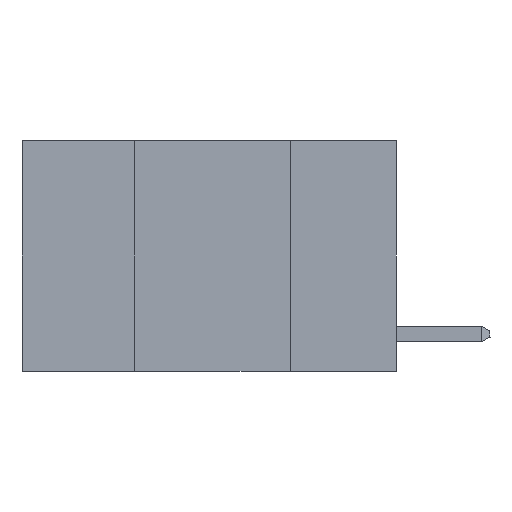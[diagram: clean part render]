
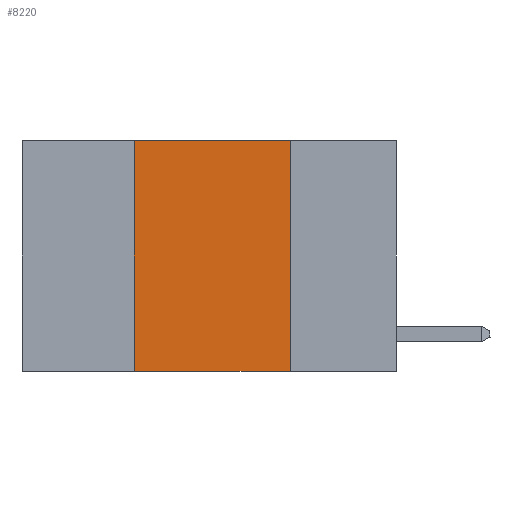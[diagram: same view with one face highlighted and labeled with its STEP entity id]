
A CAD part, left-side view. The second image highlights one B-rep face of the part: STEP entity #8220.
In plain terms, the highlighted planar face has unit normal (-1, 0, 0).
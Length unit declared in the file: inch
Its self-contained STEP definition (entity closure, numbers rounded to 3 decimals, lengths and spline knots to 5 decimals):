
#167 = CARTESIAN_POINT ( 'NONE',  ( 0., 0.6, 0. ) ) ;
#1373 = DIRECTION ( 'NONE',  ( 1., 0., 0. ) ) ;
#1791 = CARTESIAN_POINT ( 'NONE',  ( 0., 0.17, -0.37 ) ) ;
#2499 = VECTOR ( 'NONE', #4436, 39.37008 ) ;
#2745 = VERTEX_POINT ( 'NONE', #5468 ) ;
#3019 = VERTEX_POINT ( 'NONE', #10564 ) ;
#3190 = EDGE_LOOP ( 'NONE', ( #9456, #6426, #9125, #6053 ) ) ;
#3702 = FACE_OUTER_BOUND ( 'NONE', #3190, .T. ) ;
#3731 = CARTESIAN_POINT ( 'NONE',  ( 0., 0.6, 0. ) ) ;
#4072 = EDGE_CURVE ( 'NONE', #3019, #5443, #5163, .T. ) ;
#4385 = LINE ( 'NONE', #3731, #7846 ) ;
#4436 = DIRECTION ( 'NONE',  ( 0., 0., 1. ) ) ;
#4577 = VECTOR ( 'NONE', #6348, 39.37008 ) ;
#4835 = DIRECTION ( 'NONE',  ( 0., -1., 0. ) ) ;
#5163 = LINE ( 'NONE', #11333, #2499 ) ;
#5443 = VERTEX_POINT ( 'NONE', #8613 ) ;
#5468 = CARTESIAN_POINT ( 'NONE',  ( 0., 0.17, 0. ) ) ;
#6053 = ORIENTED_EDGE ( 'NONE', *, *, #10685, .T. ) ;
#6348 = DIRECTION ( 'NONE',  ( 0., 0., -1. ) ) ;
#6426 = ORIENTED_EDGE ( 'NONE', *, *, #6625, .F. ) ;
#6625 = EDGE_CURVE ( 'NONE', #5443, #2745, #4385, .T. ) ;
#7168 = PLANE ( 'NONE',  #11584 ) ;
#7846 = VECTOR ( 'NONE', #4835, 39.37008 ) ;
#8220 = ADVANCED_FACE ( 'NONE', ( #3702 ), #7168, .F. ) ;
#8472 = VERTEX_POINT ( 'NONE', #1791 ) ;
#8613 = CARTESIAN_POINT ( 'NONE',  ( 0., 0.42, 0. ) ) ;
#9125 = ORIENTED_EDGE ( 'NONE', *, *, #4072, .F. ) ;
#9431 = DIRECTION ( 'NONE',  ( 0., 0., -1. ) ) ;
#9456 = ORIENTED_EDGE ( 'NONE', *, *, #13700, .F. ) ;
#10000 = DIRECTION ( 'NONE',  ( 0., -1., 0. ) ) ;
#10357 = LINE ( 'NONE', #14441, #4577 ) ;
#10564 = CARTESIAN_POINT ( 'NONE',  ( 0., 0.42, -0.37 ) ) ;
#10651 = VECTOR ( 'NONE', #10000, 39.37008 ) ;
#10685 = EDGE_CURVE ( 'NONE', #3019, #8472, #13754, .T. ) ;
#11333 = CARTESIAN_POINT ( 'NONE',  ( 0., 0.42, 0. ) ) ;
#11584 = AXIS2_PLACEMENT_3D ( 'NONE', #167, #1373, #9431 ) ;
#13700 = EDGE_CURVE ( 'NONE', #2745, #8472, #10357, .T. ) ;
#13754 = LINE ( 'NONE', #14646, #10651 ) ;
#14441 = CARTESIAN_POINT ( 'NONE',  ( 0., 0.17, 0. ) ) ;
#14646 = CARTESIAN_POINT ( 'NONE',  ( 0., 0.6, -0.37 ) ) ;
